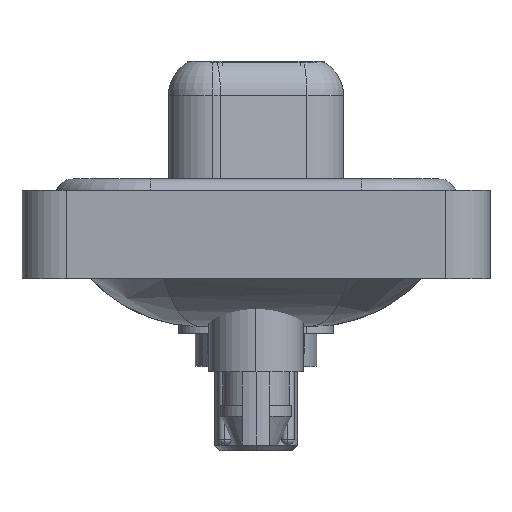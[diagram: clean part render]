
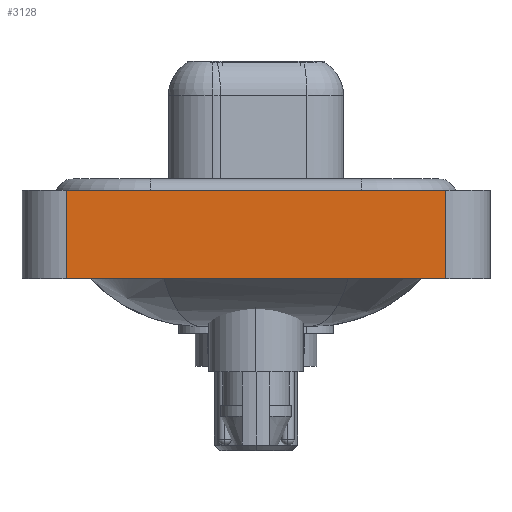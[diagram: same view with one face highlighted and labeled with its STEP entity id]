
A CAD part, left-side view. The second image highlights one B-rep face of the part: STEP entity #3128.
In plain terms, the highlighted planar face has unit normal (-1, 0, 0).
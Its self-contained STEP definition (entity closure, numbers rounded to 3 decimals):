
#556 = DIRECTION ( 'NONE',  ( -1., 0., 0. ) ) ;
#1060 = ORIENTED_EDGE ( 'NONE', *, *, #10396, .T. ) ;
#1256 = CARTESIAN_POINT ( 'NONE',  ( -7.3, -8.55, -3.6 ) ) ;
#1965 = VECTOR ( 'NONE', #13479, 1000. ) ;
#2613 = FACE_OUTER_BOUND ( 'NONE', #10265, .T. ) ;
#2851 = ORIENTED_EDGE ( 'NONE', *, *, #22582, .F. ) ;
#3128 = ADVANCED_FACE ( 'NONE', ( #2613 ), #11382, .T. ) ;
#3424 = CARTESIAN_POINT ( 'NONE',  ( -7.3, 8.55, -3.6 ) ) ;
#4714 = LINE ( 'NONE', #3424, #5228 ) ;
#5228 = VECTOR ( 'NONE', #13796, 1000. ) ;
#5774 = DIRECTION ( 'NONE',  ( 0., 0., 1. ) ) ;
#6328 = LINE ( 'NONE', #13681, #10544 ) ;
#7327 = AXIS2_PLACEMENT_3D ( 'NONE', #16486, #556, #5774 ) ;
#7694 = ORIENTED_EDGE ( 'NONE', *, *, #9303, .T. ) ;
#8501 = CARTESIAN_POINT ( 'NONE',  ( -7.3, 8.55, -3.6 ) ) ;
#8857 = CARTESIAN_POINT ( 'NONE',  ( -7.3, -8.55, 0.4 ) ) ;
#8982 = CARTESIAN_POINT ( 'NONE',  ( -7.3, -8.55, 0.4 ) ) ;
#9303 = EDGE_CURVE ( 'NONE', #13557, #13682, #17072, .T. ) ;
#10265 = EDGE_LOOP ( 'NONE', ( #7694, #2851, #11649, #1060 ) ) ;
#10396 = EDGE_CURVE ( 'NONE', #13746, #13557, #6328, .T. ) ;
#10544 = VECTOR ( 'NONE', #13454, 1000. ) ;
#10651 = CARTESIAN_POINT ( 'NONE',  ( -7.3, 8.55, 0.4 ) ) ;
#10826 = VERTEX_POINT ( 'NONE', #10651 ) ;
#11382 = PLANE ( 'NONE',  #7327 ) ;
#11649 = ORIENTED_EDGE ( 'NONE', *, *, #16233, .F. ) ;
#13454 = DIRECTION ( 'NONE',  ( 0., -1., 0. ) ) ;
#13479 = DIRECTION ( 'NONE',  ( 0., 0., 1. ) ) ;
#13557 = VERTEX_POINT ( 'NONE', #17250 ) ;
#13681 = CARTESIAN_POINT ( 'NONE',  ( -7.3, -8.55, -3.6 ) ) ;
#13682 = VERTEX_POINT ( 'NONE', #8857 ) ;
#13746 = VERTEX_POINT ( 'NONE', #8501 ) ;
#13796 = DIRECTION ( 'NONE',  ( 0., 0., 1. ) ) ;
#14001 = DIRECTION ( 'NONE',  ( 0., -1., 0. ) ) ;
#16083 = LINE ( 'NONE', #8982, #18316 ) ;
#16233 = EDGE_CURVE ( 'NONE', #13746, #10826, #4714, .T. ) ;
#16486 = CARTESIAN_POINT ( 'NONE',  ( -7.3, -8.55, -3.6 ) ) ;
#17072 = LINE ( 'NONE', #1256, #1965 ) ;
#17250 = CARTESIAN_POINT ( 'NONE',  ( -7.3, -8.55, -3.6 ) ) ;
#18316 = VECTOR ( 'NONE', #14001, 1000. ) ;
#22582 = EDGE_CURVE ( 'NONE', #10826, #13682, #16083, .T. ) ;
